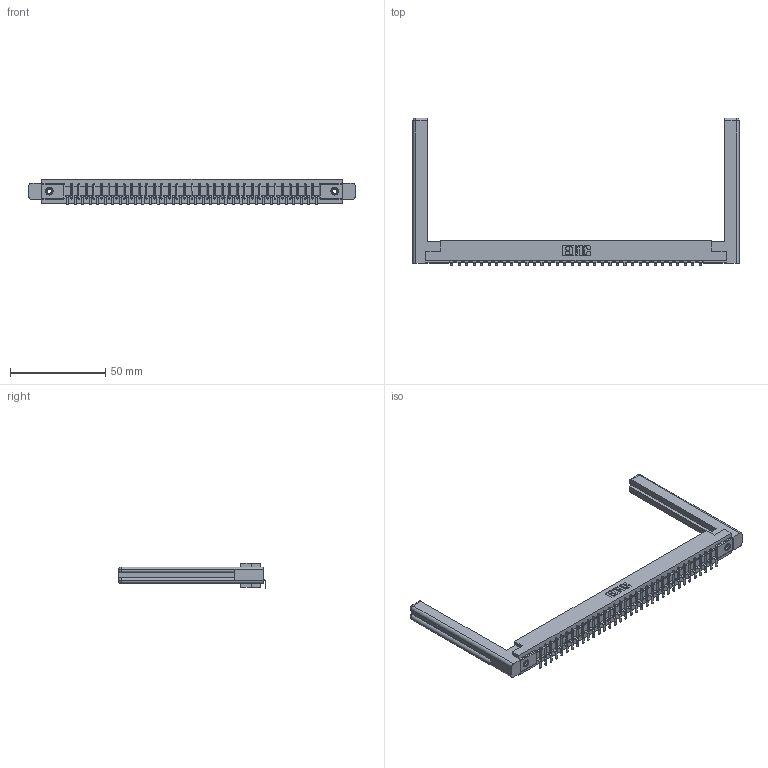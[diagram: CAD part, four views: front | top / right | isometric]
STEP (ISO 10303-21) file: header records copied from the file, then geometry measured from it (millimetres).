
FILE_DESCRIPTION (( 'STEP AP203' ), '1' );
FILE_NAME ('307-034-553-158.STEP', '2019-09-05T06:41:55', ( '' ), ( '' ), 'SwSTEP 2.0', 'SolidWorks 2016', '' );
FILE_SCHEMA (( 'CONFIG_CONTROL_DESIGN' ));
Length unit declared in the file: inch
Products named in the file (5): 307-220-058; 345-250-001_345-250-001-102; 307-290-002_553; 307-034-553-158; 307 Part_.156 Dia Mounting Holes
Assembly tree (39 placements, depth 2):
  307-034-553-158
    307 Part_.156 Dia Mounting Holes
    307-290-002_553  x34
    307-220-058  x2
    345-250-001_345-250-001-102  x2
Bounding box: 171.35 x 77.64 x 13.5 mm (x, y, z)
Volume: 25396.9 mm3; surface area: 27631.3 mm2
Topology: 39 solids, 39 shells, 2947 faces, 8973 edges, 5874 vertices
Faces by surface type: plane 1752, cylinder 1101, sphere 70, torus 12, cone 12
Entity records: 33621 total; most frequent: CARTESIAN_POINT 5679, ORIENTED_EDGE 5608, DIRECTION 5482, EDGE_CURVE 2804, VECTOR 2140, LINE 2140, VERTEX_POINT 1814, AXIS2_PLACEMENT_3D 1671
